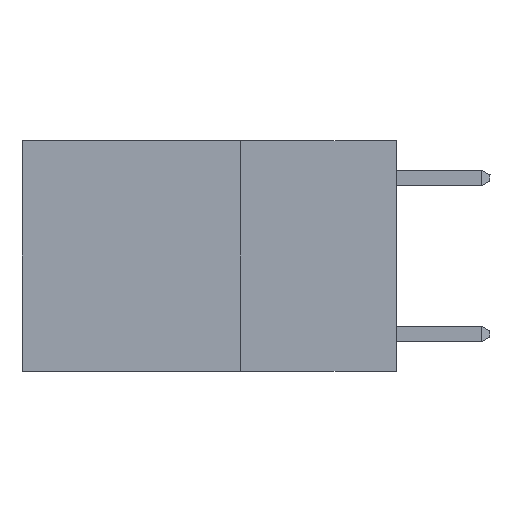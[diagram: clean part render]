
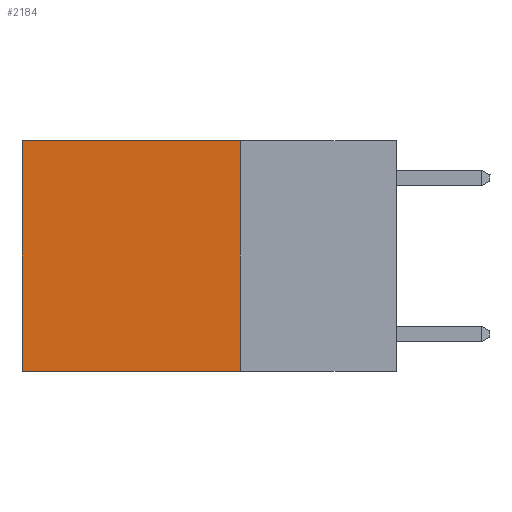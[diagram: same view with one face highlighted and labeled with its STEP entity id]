
A CAD part, left-side view. The second image highlights one B-rep face of the part: STEP entity #2184.
In plain terms, the highlighted planar face has unit normal (-1, 0, 0).
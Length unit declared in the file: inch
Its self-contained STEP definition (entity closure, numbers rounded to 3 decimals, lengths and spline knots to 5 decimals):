
#860 = LINE ( 'NONE', #14458, #14430 ) ;
#1136 = ORIENTED_EDGE ( 'NONE', *, *, #11629, .F. ) ;
#1207 = DIRECTION ( 'NONE',  ( 1., 0., 0. ) ) ;
#1222 = VECTOR ( 'NONE', #6242, 39.37008 ) ;
#1565 = ORIENTED_EDGE ( 'NONE', *, *, #9795, .F. ) ;
#2184 = ADVANCED_FACE ( 'NONE', ( #13644 ), #14959, .F. ) ;
#6242 = DIRECTION ( 'NONE',  ( 0., 1., 0. ) ) ;
#6449 = EDGE_CURVE ( 'NONE', #12193, #8909, #10566, .T. ) ;
#6622 = CARTESIAN_POINT ( 'NONE',  ( 0.2625, 0.6, 0. ) ) ;
#7386 = ORIENTED_EDGE ( 'NONE', *, *, #6449, .T. ) ;
#8026 = VERTEX_POINT ( 'NONE', #13837 ) ;
#8385 = DIRECTION ( 'NONE',  ( 0., 0., -1. ) ) ;
#8689 = VERTEX_POINT ( 'NONE', #13089 ) ;
#8909 = VERTEX_POINT ( 'NONE', #14874 ) ;
#9235 = EDGE_CURVE ( 'NONE', #8689, #12193, #860, .T. ) ;
#9343 = DIRECTION ( 'NONE',  ( 0., 0., -1. ) ) ;
#9612 = EDGE_LOOP ( 'NONE', ( #7386, #1136, #1565, #16158 ) ) ;
#9795 = EDGE_CURVE ( 'NONE', #8689, #8026, #14831, .T. ) ;
#10026 = CARTESIAN_POINT ( 'NONE',  ( 0.2625, 0.25, -0.37 ) ) ;
#10566 = LINE ( 'NONE', #15481, #11448 ) ;
#10831 = CARTESIAN_POINT ( 'NONE',  ( 0.2625, 0.25, 0. ) ) ;
#11448 = VECTOR ( 'NONE', #9343, 39.37008 ) ;
#11629 = EDGE_CURVE ( 'NONE', #8026, #8909, #15088, .T. ) ;
#12193 = VERTEX_POINT ( 'NONE', #6622 ) ;
#12420 = CARTESIAN_POINT ( 'NONE',  ( 0.2625, 0.25, 0. ) ) ;
#12619 = VECTOR ( 'NONE', #8385, 39.37008 ) ;
#13089 = CARTESIAN_POINT ( 'NONE',  ( 0.2625, 0.25, 0. ) ) ;
#13557 = DIRECTION ( 'NONE',  ( 0., 0., -1. ) ) ;
#13644 = FACE_OUTER_BOUND ( 'NONE', #9612, .T. ) ;
#13837 = CARTESIAN_POINT ( 'NONE',  ( 0.2625, 0.25, -0.37 ) ) ;
#14430 = VECTOR ( 'NONE', #15790, 39.37008 ) ;
#14458 = CARTESIAN_POINT ( 'NONE',  ( 0.2625, 0.25, 0. ) ) ;
#14831 = LINE ( 'NONE', #10831, #12619 ) ;
#14874 = CARTESIAN_POINT ( 'NONE',  ( 0.2625, 0.6, -0.37 ) ) ;
#14959 = PLANE ( 'NONE',  #15035 ) ;
#15035 = AXIS2_PLACEMENT_3D ( 'NONE', #12420, #1207, #13557 ) ;
#15088 = LINE ( 'NONE', #10026, #1222 ) ;
#15481 = CARTESIAN_POINT ( 'NONE',  ( 0.2625, 0.6, 0. ) ) ;
#15790 = DIRECTION ( 'NONE',  ( 0., 1., 0. ) ) ;
#16158 = ORIENTED_EDGE ( 'NONE', *, *, #9235, .T. ) ;
